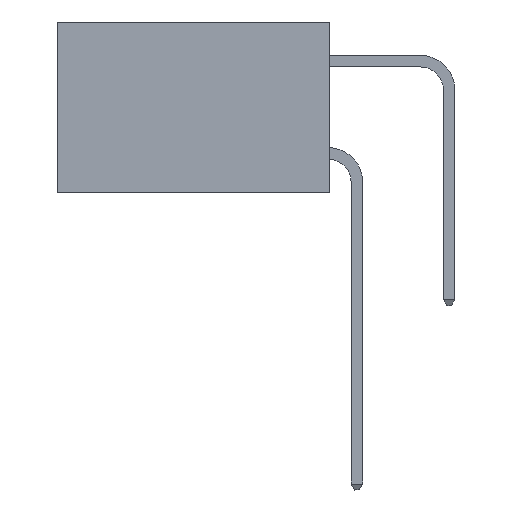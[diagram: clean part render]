
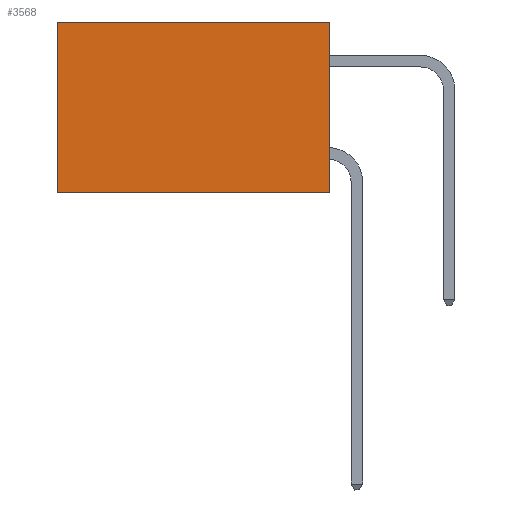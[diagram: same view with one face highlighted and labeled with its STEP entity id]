
A CAD part, left-side view. The second image highlights one B-rep face of the part: STEP entity #3568.
In plain terms, the highlighted planar face has unit normal (-1, 0, 0).
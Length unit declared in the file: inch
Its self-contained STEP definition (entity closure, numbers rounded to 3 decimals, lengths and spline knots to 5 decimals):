
#1298 = VERTEX_POINT ( 'NONE', #14557 ) ;
#1689 = CARTESIAN_POINT ( 'NONE',  ( 0.277, 0.59, -0.37 ) ) ;
#1699 = EDGE_CURVE ( 'NONE', #12099, #1298, #18447, .T. ) ;
#1806 = CARTESIAN_POINT ( 'NONE',  ( 0.277, 0., -0.37 ) ) ;
#1997 = LINE ( 'NONE', #1689, #11879 ) ;
#2027 = DIRECTION ( 'NONE',  ( 0., 0., -1. ) ) ;
#2477 = EDGE_CURVE ( 'NONE', #16735, #9895, #1997, .T. ) ;
#3568 = ADVANCED_FACE ( 'NONE', ( #22885 ), #23539, .F. ) ;
#4133 = CARTESIAN_POINT ( 'NONE',  ( 0.277, 0.59, -0.37 ) ) ;
#5637 = VECTOR ( 'NONE', #6983, 39.37008 ) ;
#6983 = DIRECTION ( 'NONE',  ( 0., 1., 0. ) ) ;
#6988 = ORIENTED_EDGE ( 'NONE', *, *, #1699, .F. ) ;
#7979 = ORIENTED_EDGE ( 'NONE', *, *, #21691, .F. ) ;
#9895 = VERTEX_POINT ( 'NONE', #4133 ) ;
#10250 = CARTESIAN_POINT ( 'NONE',  ( 0.277, 0.59, 0. ) ) ;
#11462 = DIRECTION ( 'NONE',  ( 0., 0., -1. ) ) ;
#11842 = CARTESIAN_POINT ( 'NONE',  ( 0.277, 0., -0.37 ) ) ;
#11879 = VECTOR ( 'NONE', #2027, 39.37008 ) ;
#12099 = VERTEX_POINT ( 'NONE', #17237 ) ;
#13286 = ORIENTED_EDGE ( 'NONE', *, *, #16730, .T. ) ;
#14312 = CARTESIAN_POINT ( 'NONE',  ( 0.277, 0., -0.37 ) ) ;
#14557 = CARTESIAN_POINT ( 'NONE',  ( 0.277, 0., -0.37 ) ) ;
#16730 = EDGE_CURVE ( 'NONE', #12099, #16735, #22071, .T. ) ;
#16735 = VERTEX_POINT ( 'NONE', #10250 ) ;
#17237 = CARTESIAN_POINT ( 'NONE',  ( 0.277, 0., 0. ) ) ;
#17280 = VECTOR ( 'NONE', #19349, 39.37008 ) ;
#17514 = CARTESIAN_POINT ( 'NONE',  ( 0.277, 0., 0. ) ) ;
#18196 = VECTOR ( 'NONE', #11462, 39.37008 ) ;
#18322 = ORIENTED_EDGE ( 'NONE', *, *, #2477, .T. ) ;
#18442 = EDGE_LOOP ( 'NONE', ( #18322, #7979, #6988, #13286 ) ) ;
#18447 = LINE ( 'NONE', #1806, #18196 ) ;
#19349 = DIRECTION ( 'NONE',  ( 0., 1., 0. ) ) ;
#20789 = LINE ( 'NONE', #14312, #5637 ) ;
#21691 = EDGE_CURVE ( 'NONE', #1298, #9895, #20789, .T. ) ;
#22071 = LINE ( 'NONE', #17514, #17280 ) ;
#22885 = FACE_OUTER_BOUND ( 'NONE', #18442, .T. ) ;
#23097 = AXIS2_PLACEMENT_3D ( 'NONE', #11842, #23520, #23496 ) ;
#23496 = DIRECTION ( 'NONE',  ( 0., 0., -1. ) ) ;
#23520 = DIRECTION ( 'NONE',  ( 1., 0., 0. ) ) ;
#23539 = PLANE ( 'NONE',  #23097 ) ;
